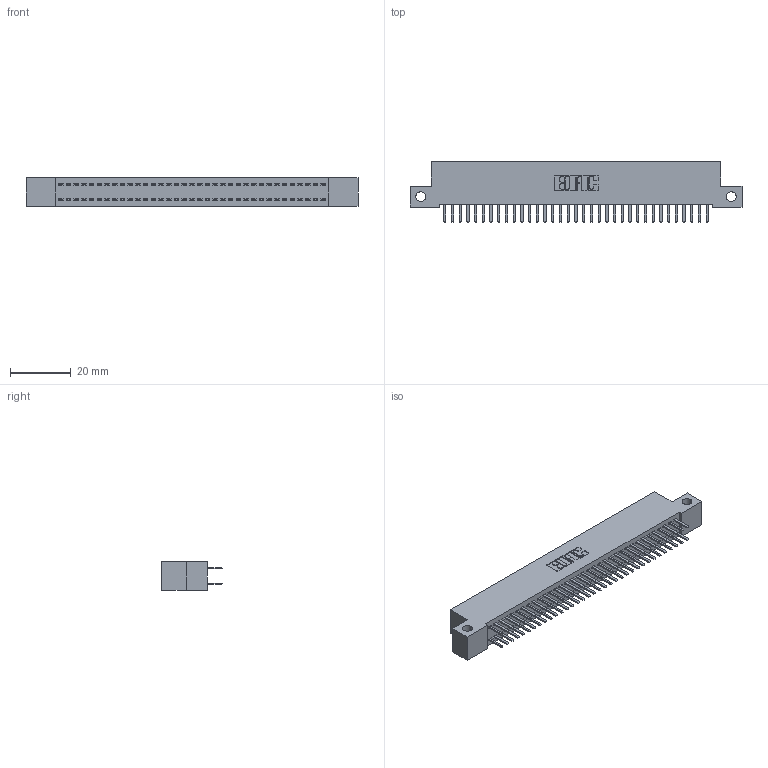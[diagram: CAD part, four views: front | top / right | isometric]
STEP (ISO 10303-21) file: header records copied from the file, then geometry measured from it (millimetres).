
FILE_DESCRIPTION (( 'STEP AP203' ), '1' );
FILE_NAME ('392-070-520-212.STEP', '2019-10-09T11:56:39', ( '' ), ( '' ), 'SwSTEP 2.0', 'SolidWorks 2016', '' );
FILE_SCHEMA (( 'CONFIG_CONTROL_DESIGN' ));
Length unit declared in the file: inch
Products named in the file (3): 345-292-001_345-293-120; 392-070-520-212; 342 Part_Side Mount
Assembly tree (71 placements, depth 2):
  392-070-520-212
    342 Part_Side Mount
    345-292-001_345-293-120  x70
Bounding box: 109.22 x 20.02 x 9.4 mm (x, y, z)
Volume: 9675.6 mm3; surface area: 15344.6 mm2
Topology: 71 solids, 71 shells, 4030 faces, 11709 edges, 7618 vertices
Faces by surface type: plane 2726, cylinder 1304
Entity records: 23407 total; most frequent: CARTESIAN_POINT 3898, ORIENTED_EDGE 3822, DIRECTION 3331, EDGE_CURVE 1911, LINE 1779, VECTOR 1779, VERTEX_POINT 1270, AXIS2_PLACEMENT_3D 776
